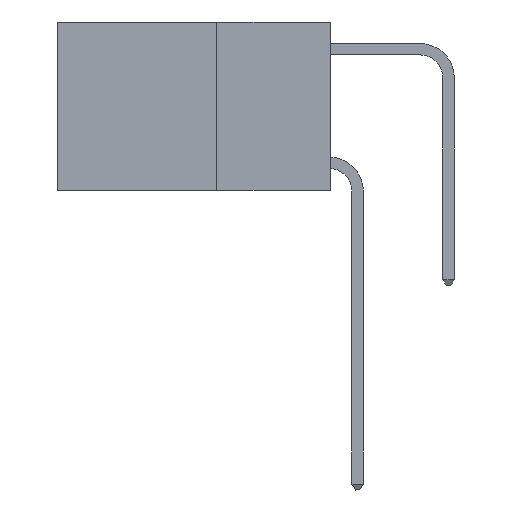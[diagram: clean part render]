
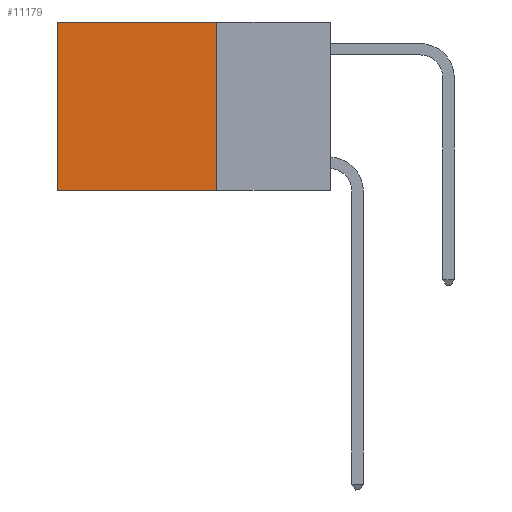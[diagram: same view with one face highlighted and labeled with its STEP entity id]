
A CAD part, left-side view. The second image highlights one B-rep face of the part: STEP entity #11179.
In plain terms, the highlighted planar face has unit normal (-1, 0, 0).
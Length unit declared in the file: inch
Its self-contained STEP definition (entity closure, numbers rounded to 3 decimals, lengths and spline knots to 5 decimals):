
#190 = EDGE_CURVE ( 'NONE', #2669, #4030, #4666, .T. ) ;
#319 = EDGE_CURVE ( 'NONE', #3365, #2669, #12983, .T. ) ;
#378 = CARTESIAN_POINT ( 'NONE',  ( 0.2625, 0.25, -0.37 ) ) ;
#432 = DIRECTION ( 'NONE',  ( 0., 0., -1. ) ) ;
#490 = VECTOR ( 'NONE', #6189, 39.37008 ) ;
#511 = CARTESIAN_POINT ( 'NONE',  ( 0.2625, 0.6, -0.37 ) ) ;
#1719 = CARTESIAN_POINT ( 'NONE',  ( 0.2625, 0.25, 0. ) ) ;
#2146 = DIRECTION ( 'NONE',  ( 0., 0., -1. ) ) ;
#2151 = CARTESIAN_POINT ( 'NONE',  ( 0.2625, 0.25, 0. ) ) ;
#2512 = FACE_OUTER_BOUND ( 'NONE', #8969, .T. ) ;
#2669 = VERTEX_POINT ( 'NONE', #5565 ) ;
#2805 = DIRECTION ( 'NONE',  ( 0., 0., -1. ) ) ;
#3365 = VERTEX_POINT ( 'NONE', #7909 ) ;
#3444 = LINE ( 'NONE', #4228, #6127 ) ;
#3597 = ORIENTED_EDGE ( 'NONE', *, *, #10186, .F. ) ;
#4030 = VERTEX_POINT ( 'NONE', #511 ) ;
#4053 = ORIENTED_EDGE ( 'NONE', *, *, #319, .T. ) ;
#4228 = CARTESIAN_POINT ( 'NONE',  ( 0.2625, 0.25, 0. ) ) ;
#4529 = CARTESIAN_POINT ( 'NONE',  ( 0.2625, 0.25, -0.37 ) ) ;
#4666 = LINE ( 'NONE', #8507, #10199 ) ;
#5565 = CARTESIAN_POINT ( 'NONE',  ( 0.2625, 0.6, 0. ) ) ;
#5722 = VERTEX_POINT ( 'NONE', #378 ) ;
#6127 = VECTOR ( 'NONE', #2146, 39.37008 ) ;
#6189 = DIRECTION ( 'NONE',  ( 0., 1., 0. ) ) ;
#7909 = CARTESIAN_POINT ( 'NONE',  ( 0.2625, 0.25, 0. ) ) ;
#8244 = AXIS2_PLACEMENT_3D ( 'NONE', #1719, #8749, #2805 ) ;
#8507 = CARTESIAN_POINT ( 'NONE',  ( 0.2625, 0.6, 0. ) ) ;
#8749 = DIRECTION ( 'NONE',  ( 1., 0., 0. ) ) ;
#8969 = EDGE_LOOP ( 'NONE', ( #10310, #9986, #3597, #4053 ) ) ;
#9412 = DIRECTION ( 'NONE',  ( 0., 1., 0. ) ) ;
#9986 = ORIENTED_EDGE ( 'NONE', *, *, #12357, .F. ) ;
#10186 = EDGE_CURVE ( 'NONE', #3365, #5722, #3444, .T. ) ;
#10199 = VECTOR ( 'NONE', #432, 39.37008 ) ;
#10258 = VECTOR ( 'NONE', #9412, 39.37008 ) ;
#10310 = ORIENTED_EDGE ( 'NONE', *, *, #190, .T. ) ;
#10704 = PLANE ( 'NONE',  #8244 ) ;
#11179 = ADVANCED_FACE ( 'NONE', ( #2512 ), #10704, .F. ) ;
#12357 = EDGE_CURVE ( 'NONE', #5722, #4030, #12894, .T. ) ;
#12894 = LINE ( 'NONE', #4529, #10258 ) ;
#12983 = LINE ( 'NONE', #2151, #490 ) ;
